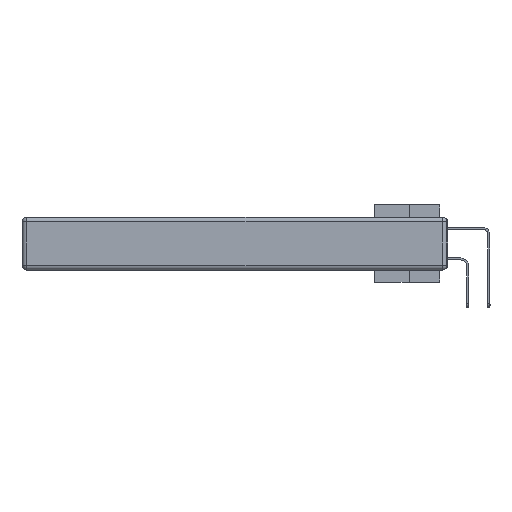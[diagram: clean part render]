
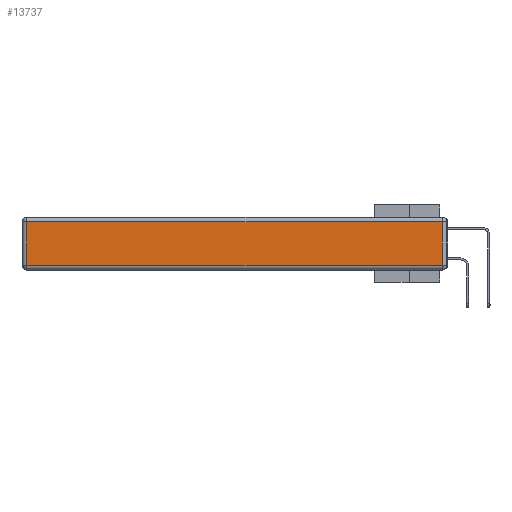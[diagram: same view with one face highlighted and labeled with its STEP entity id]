
A CAD part, left-side view. The second image highlights one B-rep face of the part: STEP entity #13737.
In plain terms, the highlighted planar face has unit normal (-1, 0, 0).
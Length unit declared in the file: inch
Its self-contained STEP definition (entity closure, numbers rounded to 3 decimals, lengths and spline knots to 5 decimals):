
#216 = EDGE_CURVE ( 'NONE', #16820, #24788, #32379, .T. ) ;
#2588 = CARTESIAN_POINT ( 'NONE',  ( 0., 2.72, -0.03 ) ) ;
#2670 = EDGE_LOOP ( 'NONE', ( #32763, #26338, #16710, #14422 ) ) ;
#3821 = FACE_OUTER_BOUND ( 'NONE', #2670, .T. ) ;
#5574 = DIRECTION ( 'NONE',  ( 0., 0., 1. ) ) ;
#7537 = PLANE ( 'NONE',  #36997 ) ;
#8355 = CARTESIAN_POINT ( 'NONE',  ( 0., 0.03, -0.03 ) ) ;
#8847 = DIRECTION ( 'NONE',  ( 0., 0., -1. ) ) ;
#10493 = CARTESIAN_POINT ( 'NONE',  ( 0., 2.72, -0.313 ) ) ;
#10617 = DIRECTION ( 'NONE',  ( -1., 0., 0. ) ) ;
#12193 = CARTESIAN_POINT ( 'NONE',  ( 0., 2.75, -0.03 ) ) ;
#12380 = VERTEX_POINT ( 'NONE', #10493 ) ;
#12831 = LINE ( 'NONE', #12193, #15228 ) ;
#13672 = VECTOR ( 'NONE', #8847, 39.37008 ) ;
#13737 = ADVANCED_FACE ( 'NONE', ( #3821 ), #7537, .T. ) ;
#14422 = ORIENTED_EDGE ( 'NONE', *, *, #16019, .T. ) ;
#15228 = VECTOR ( 'NONE', #33777, 39.37008 ) ;
#16019 = EDGE_CURVE ( 'NONE', #21613, #12380, #29795, .T. ) ;
#16710 = ORIENTED_EDGE ( 'NONE', *, *, #20553, .T. ) ;
#16820 = VERTEX_POINT ( 'NONE', #25542 ) ;
#17644 = CARTESIAN_POINT ( 'NONE',  ( 0., 2.72, -0.343 ) ) ;
#20553 = EDGE_CURVE ( 'NONE', #24788, #21613, #12831, .T. ) ;
#21613 = VERTEX_POINT ( 'NONE', #2588 ) ;
#22856 = VECTOR ( 'NONE', #27095, 39.37008 ) ;
#24788 = VERTEX_POINT ( 'NONE', #8355 ) ;
#25525 = DIRECTION ( 'NONE',  ( 0., 0., 1. ) ) ;
#25542 = CARTESIAN_POINT ( 'NONE',  ( 0., 0.03, -0.313 ) ) ;
#26081 = CARTESIAN_POINT ( 'NONE',  ( 0., 0.03, -0.343 ) ) ;
#26338 = ORIENTED_EDGE ( 'NONE', *, *, #216, .T. ) ;
#27095 = DIRECTION ( 'NONE',  ( 0., -1., 0. ) ) ;
#28528 = VECTOR ( 'NONE', #25525, 39.37008 ) ;
#28745 = CARTESIAN_POINT ( 'NONE',  ( 0., 0., -0.343 ) ) ;
#29795 = LINE ( 'NONE', #17644, #13672 ) ;
#29971 = LINE ( 'NONE', #35850, #22856 ) ;
#32379 = LINE ( 'NONE', #26081, #28528 ) ;
#32763 = ORIENTED_EDGE ( 'NONE', *, *, #37749, .T. ) ;
#33777 = DIRECTION ( 'NONE',  ( 0., 1., 0. ) ) ;
#35850 = CARTESIAN_POINT ( 'NONE',  ( 0., 0., -0.313 ) ) ;
#36997 = AXIS2_PLACEMENT_3D ( 'NONE', #28745, #10617, #5574 ) ;
#37749 = EDGE_CURVE ( 'NONE', #12380, #16820, #29971, .T. ) ;
